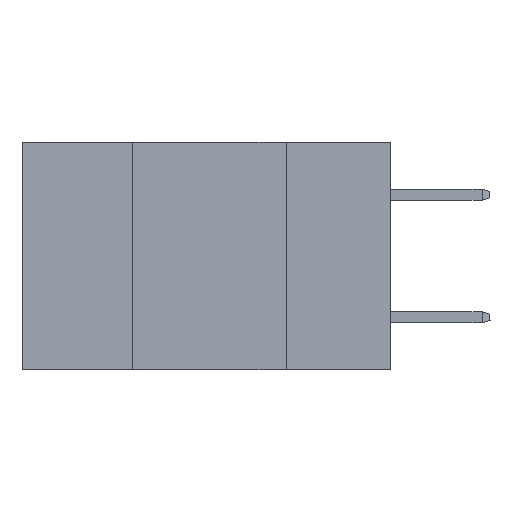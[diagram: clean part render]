
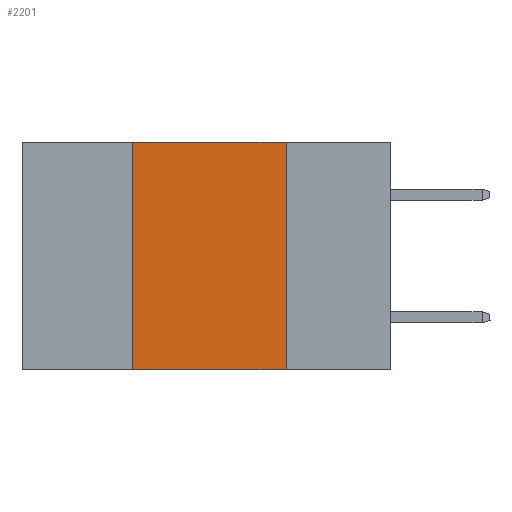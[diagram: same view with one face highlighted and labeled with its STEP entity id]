
A CAD part, left-side view. The second image highlights one B-rep face of the part: STEP entity #2201.
In plain terms, the highlighted planar face has unit normal (-1, 0, 0).
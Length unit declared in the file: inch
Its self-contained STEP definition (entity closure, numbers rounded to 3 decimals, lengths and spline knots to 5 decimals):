
#413 = DIRECTION ( 'NONE',  ( 0., 0., 1. ) ) ;
#820 = EDGE_CURVE ( 'NONE', #17621, #8453, #4992, .T. ) ;
#1360 = PLANE ( 'NONE',  #11514 ) ;
#2201 = ADVANCED_FACE ( 'NONE', ( #9073 ), #1360, .F. ) ;
#2520 = CARTESIAN_POINT ( 'NONE',  ( 0., 0.6, 0. ) ) ;
#2596 = CARTESIAN_POINT ( 'NONE',  ( 0., 0.17, 0. ) ) ;
#2650 = VECTOR ( 'NONE', #413, 39.37008 ) ;
#3449 = CARTESIAN_POINT ( 'NONE',  ( 0., 0.42, -0.37 ) ) ;
#3814 = DIRECTION ( 'NONE',  ( 0., -1., 0. ) ) ;
#3924 = DIRECTION ( 'NONE',  ( 0., 0., -1. ) ) ;
#4024 = ORIENTED_EDGE ( 'NONE', *, *, #4122, .F. ) ;
#4122 = EDGE_CURVE ( 'NONE', #7214, #8453, #7688, .T. ) ;
#4992 = LINE ( 'NONE', #16261, #10359 ) ;
#5257 = EDGE_CURVE ( 'NONE', #17621, #14371, #6147, .T. ) ;
#5985 = ORIENTED_EDGE ( 'NONE', *, *, #5257, .F. ) ;
#6147 = LINE ( 'NONE', #15722, #2650 ) ;
#7214 = VERTEX_POINT ( 'NONE', #11832 ) ;
#7688 = LINE ( 'NONE', #2596, #11799 ) ;
#8113 = DIRECTION ( 'NONE',  ( 0., 0., -1. ) ) ;
#8453 = VERTEX_POINT ( 'NONE', #17137 ) ;
#8685 = VECTOR ( 'NONE', #10600, 39.37008 ) ;
#9073 = FACE_OUTER_BOUND ( 'NONE', #9213, .T. ) ;
#9213 = EDGE_LOOP ( 'NONE', ( #4024, #14663, #5985, #12798 ) ) ;
#9225 = CARTESIAN_POINT ( 'NONE',  ( 0., 0.6, 0. ) ) ;
#10359 = VECTOR ( 'NONE', #3814, 39.37008 ) ;
#10600 = DIRECTION ( 'NONE',  ( 0., -1., 0. ) ) ;
#11514 = AXIS2_PLACEMENT_3D ( 'NONE', #2520, #15082, #3924 ) ;
#11799 = VECTOR ( 'NONE', #8113, 39.37008 ) ;
#11832 = CARTESIAN_POINT ( 'NONE',  ( 0., 0.17, 0. ) ) ;
#12798 = ORIENTED_EDGE ( 'NONE', *, *, #820, .T. ) ;
#13534 = EDGE_CURVE ( 'NONE', #14371, #7214, #14386, .T. ) ;
#14371 = VERTEX_POINT ( 'NONE', #18014 ) ;
#14386 = LINE ( 'NONE', #9225, #8685 ) ;
#14663 = ORIENTED_EDGE ( 'NONE', *, *, #13534, .F. ) ;
#15082 = DIRECTION ( 'NONE',  ( 1., 0., 0. ) ) ;
#15722 = CARTESIAN_POINT ( 'NONE',  ( 0., 0.42, 0. ) ) ;
#16261 = CARTESIAN_POINT ( 'NONE',  ( 0., 0.6, -0.37 ) ) ;
#17137 = CARTESIAN_POINT ( 'NONE',  ( 0., 0.17, -0.37 ) ) ;
#17621 = VERTEX_POINT ( 'NONE', #3449 ) ;
#18014 = CARTESIAN_POINT ( 'NONE',  ( 0., 0.42, 0. ) ) ;
